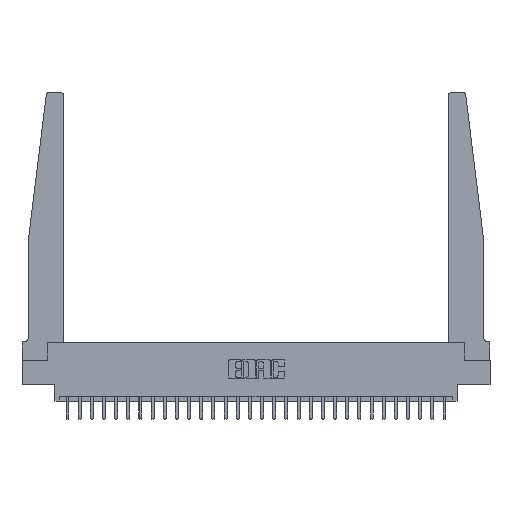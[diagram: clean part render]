
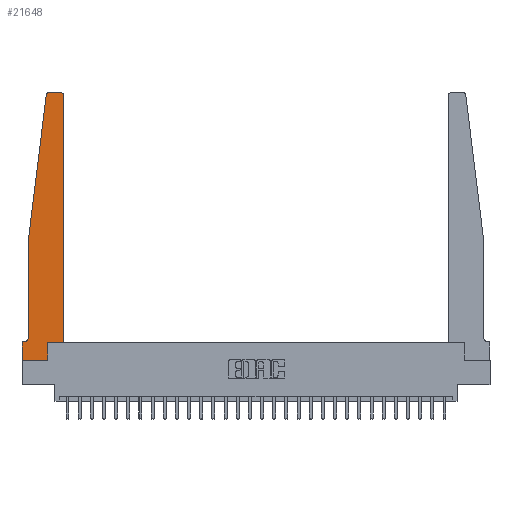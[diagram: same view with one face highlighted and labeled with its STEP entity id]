
A CAD part, top view. The second image highlights one B-rep face of the part: STEP entity #21648.
In plain terms, the highlighted planar face has unit normal (0, 0, 1).
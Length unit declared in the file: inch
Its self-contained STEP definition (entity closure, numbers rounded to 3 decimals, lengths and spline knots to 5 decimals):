
#173 = DIRECTION ( 'NONE',  ( 0., 0., 1. ) ) ;
#716 = ORIENTED_EDGE ( 'NONE', *, *, #9396, .T. ) ;
#854 = CARTESIAN_POINT ( 'NONE',  ( 0.015, 0.1875, 0.37 ) ) ;
#1116 = EDGE_CURVE ( 'NONE', #3473, #13060, #21672, .T. ) ;
#1204 = CARTESIAN_POINT ( 'NONE',  ( 0.425, 0.18, 0.37 ) ) ;
#1271 = DIRECTION ( 'NONE',  ( 0., 0., 1. ) ) ;
#1339 = PLANE ( 'NONE',  #24150 ) ;
#1823 = DIRECTION ( 'NONE',  ( 1., 0., 0. ) ) ;
#2482 = CARTESIAN_POINT ( 'NONE',  ( 0.25, 2.75, 0.37 ) ) ;
#2562 = DIRECTION ( 'NONE',  ( 1., 0., 0. ) ) ;
#2970 = LINE ( 'NONE', #22010, #13400 ) ;
#3394 = CARTESIAN_POINT ( 'NONE',  ( 0.395, 2.72, 0.37 ) ) ;
#3423 = DIRECTION ( 'NONE',  ( 0., 0., -1. ) ) ;
#3473 = VERTEX_POINT ( 'NONE', #10091 ) ;
#3628 = AXIS2_PLACEMENT_3D ( 'NONE', #26942, #3423, #6823 ) ;
#3664 = DIRECTION ( 'NONE',  ( -1., 0., 0. ) ) ;
#3706 = ORIENTED_EDGE ( 'NONE', *, *, #26944, .T. ) ;
#4181 = VERTEX_POINT ( 'NONE', #7451 ) ;
#4374 = VERTEX_POINT ( 'NONE', #9113 ) ;
#4643 = ORIENTED_EDGE ( 'NONE', *, *, #26236, .T. ) ;
#5017 = DIRECTION ( 'NONE',  ( 0., -1., 0. ) ) ;
#5651 = VERTEX_POINT ( 'NONE', #7875 ) ;
#6157 = LINE ( 'NONE', #22957, #14341 ) ;
#6189 = EDGE_CURVE ( 'NONE', #23888, #14380, #6157, .T. ) ;
#6823 = DIRECTION ( 'NONE',  ( -1., 0., 0. ) ) ;
#7451 = CARTESIAN_POINT ( 'NONE',  ( 0.395, 2.75, 0.37 ) ) ;
#7567 = DIRECTION ( 'NONE',  ( 1., 0., 0. ) ) ;
#7636 = DIRECTION ( 'NONE',  ( 1., 0., 0. ) ) ;
#7875 = CARTESIAN_POINT ( 'NONE',  ( 0.2605, 0.18, 0.37 ) ) ;
#8265 = EDGE_LOOP ( 'NONE', ( #21581, #26319, #17737, #3706, #18715, #9252, #20167, #13757, #4643, #15794, #716, #25532 ) ) ;
#8805 = LINE ( 'NONE', #2482, #11767 ) ;
#9066 = LINE ( 'NONE', #13294, #14898 ) ;
#9113 = CARTESIAN_POINT ( 'NONE',  ( 0.425, 0.18, 0.37 ) ) ;
#9252 = ORIENTED_EDGE ( 'NONE', *, *, #15738, .T. ) ;
#9396 = EDGE_CURVE ( 'NONE', #4374, #24445, #24461, .T. ) ;
#9480 = FACE_OUTER_BOUND ( 'NONE', #8265, .T. ) ;
#9715 = EDGE_CURVE ( 'NONE', #13060, #23802, #15487, .T. ) ;
#10091 = CARTESIAN_POINT ( 'NONE',  ( 0.27653, 2.75, 0.37 ) ) ;
#10294 = VERTEX_POINT ( 'NONE', #854 ) ;
#10391 = VECTOR ( 'NONE', #14126, 39.37008 ) ;
#10858 = CARTESIAN_POINT ( 'NONE',  ( 0.27653, 2.72, 0.37 ) ) ;
#11767 = VECTOR ( 'NONE', #26284, 39.37008 ) ;
#12774 = CARTESIAN_POINT ( 'NONE',  ( 0.425, 2.72, 0.37 ) ) ;
#13060 = VERTEX_POINT ( 'NONE', #17174 ) ;
#13108 = CARTESIAN_POINT ( 'NONE',  ( 0.065, 1.25, 0.37 ) ) ;
#13294 = CARTESIAN_POINT ( 'NONE',  ( 0.065, 1.25, 0.37 ) ) ;
#13400 = VECTOR ( 'NONE', #7567, 39.37008 ) ;
#13502 = VECTOR ( 'NONE', #15954, 39.37008 ) ;
#13589 = DIRECTION ( 'NONE',  ( 1., 0., 0. ) ) ;
#13757 = ORIENTED_EDGE ( 'NONE', *, *, #22472, .T. ) ;
#14126 = DIRECTION ( 'NONE',  ( 0., 1., 0. ) ) ;
#14185 = CARTESIAN_POINT ( 'NONE',  ( 0.065, 0.1875, 0.37 ) ) ;
#14241 = EDGE_CURVE ( 'NONE', #5651, #4374, #17934, .T. ) ;
#14341 = VECTOR ( 'NONE', #21016, 39.37008 ) ;
#14380 = VERTEX_POINT ( 'NONE', #24911 ) ;
#14898 = VECTOR ( 'NONE', #5017, 39.37008 ) ;
#14900 = CARTESIAN_POINT ( 'NONE',  ( 0.2605, 0., 0.37 ) ) ;
#15397 = CARTESIAN_POINT ( 'NONE',  ( 0.065, 0.2375, 0.37 ) ) ;
#15428 = AXIS2_PLACEMENT_3D ( 'NONE', #10858, #173, #2562 ) ;
#15487 = LINE ( 'NONE', #13108, #25119 ) ;
#15731 = CIRCLE ( 'NONE', #3628, 0.05 ) ;
#15738 = EDGE_CURVE ( 'NONE', #10294, #23888, #22841, .T. ) ;
#15771 = DIRECTION ( 'NONE',  ( -0.122, -0.992, 0. ) ) ;
#15794 = ORIENTED_EDGE ( 'NONE', *, *, #14241, .T. ) ;
#15954 = DIRECTION ( 'NONE',  ( 0., 1., 0. ) ) ;
#16347 = VECTOR ( 'NONE', #3664, 39.37008 ) ;
#17174 = CARTESIAN_POINT ( 'NONE',  ( 0.24675, 2.72367, 0.37 ) ) ;
#17737 = ORIENTED_EDGE ( 'NONE', *, *, #9715, .T. ) ;
#17747 = VERTEX_POINT ( 'NONE', #15397 ) ;
#17934 = LINE ( 'NONE', #24354, #22063 ) ;
#18694 = CARTESIAN_POINT ( 'NONE',  ( 0.065, 1.25, 0.37 ) ) ;
#18715 = ORIENTED_EDGE ( 'NONE', *, *, #24916, .T. ) ;
#20167 = ORIENTED_EDGE ( 'NONE', *, *, #6189, .T. ) ;
#21016 = DIRECTION ( 'NONE',  ( 0., -1., 0. ) ) ;
#21064 = CARTESIAN_POINT ( 'NONE',  ( 0., 0.1875, 0.37 ) ) ;
#21581 = ORIENTED_EDGE ( 'NONE', *, *, #26937, .T. ) ;
#21648 = ADVANCED_FACE ( 'NONE', ( #9480 ), #1339, .T. ) ;
#21672 = CIRCLE ( 'NONE', #15428, 0.03 ) ;
#22010 = CARTESIAN_POINT ( 'NONE',  ( 0., 0., 0.37 ) ) ;
#22063 = VECTOR ( 'NONE', #13589, 39.37008 ) ;
#22355 = CARTESIAN_POINT ( 'NONE',  ( 0., 0.1875, 0.37 ) ) ;
#22472 = EDGE_CURVE ( 'NONE', #14380, #22909, #2970, .T. ) ;
#22841 = LINE ( 'NONE', #14185, #16347 ) ;
#22909 = VERTEX_POINT ( 'NONE', #14900 ) ;
#22957 = CARTESIAN_POINT ( 'NONE',  ( 0., 0., 0.37 ) ) ;
#23718 = CIRCLE ( 'NONE', #27314, 0.03 ) ;
#23802 = VERTEX_POINT ( 'NONE', #18694 ) ;
#23888 = VERTEX_POINT ( 'NONE', #21064 ) ;
#24150 = AXIS2_PLACEMENT_3D ( 'NONE', #22355, #26971, #7636 ) ;
#24354 = CARTESIAN_POINT ( 'NONE',  ( 0.425, 0.18, 0.37 ) ) ;
#24368 = EDGE_CURVE ( 'NONE', #24445, #4181, #23718, .T. ) ;
#24445 = VERTEX_POINT ( 'NONE', #12774 ) ;
#24461 = LINE ( 'NONE', #1204, #13502 ) ;
#24615 = LINE ( 'NONE', #25031, #10391 ) ;
#24911 = CARTESIAN_POINT ( 'NONE',  ( 0., 0., 0.37 ) ) ;
#24916 = EDGE_CURVE ( 'NONE', #17747, #10294, #15731, .T. ) ;
#25031 = CARTESIAN_POINT ( 'NONE',  ( 0.2605, 0.18, 0.37 ) ) ;
#25119 = VECTOR ( 'NONE', #15771, 39.37008 ) ;
#25532 = ORIENTED_EDGE ( 'NONE', *, *, #24368, .T. ) ;
#26236 = EDGE_CURVE ( 'NONE', #22909, #5651, #24615, .T. ) ;
#26284 = DIRECTION ( 'NONE',  ( -1., 0., 0. ) ) ;
#26319 = ORIENTED_EDGE ( 'NONE', *, *, #1116, .T. ) ;
#26937 = EDGE_CURVE ( 'NONE', #4181, #3473, #8805, .T. ) ;
#26942 = CARTESIAN_POINT ( 'NONE',  ( 0.015, 0.2375, 0.37 ) ) ;
#26944 = EDGE_CURVE ( 'NONE', #23802, #17747, #9066, .T. ) ;
#26971 = DIRECTION ( 'NONE',  ( 0., 0., 1. ) ) ;
#27314 = AXIS2_PLACEMENT_3D ( 'NONE', #3394, #1271, #1823 ) ;
